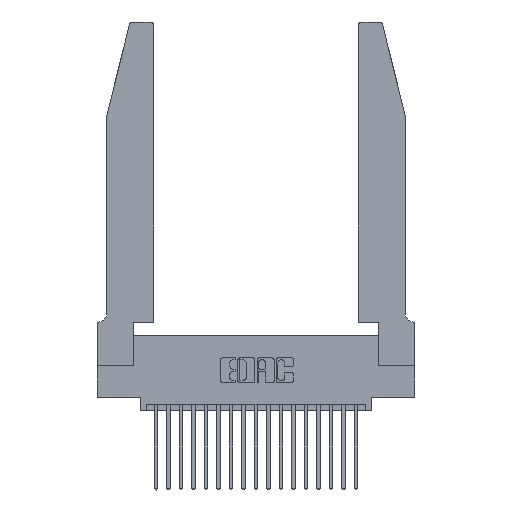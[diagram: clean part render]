
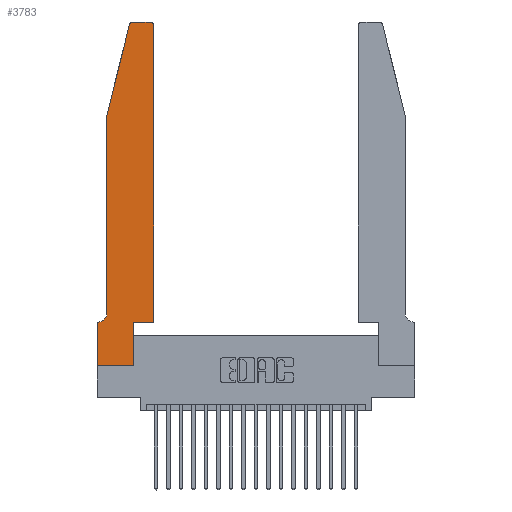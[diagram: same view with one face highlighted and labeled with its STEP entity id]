
A CAD part, top view. The second image highlights one B-rep face of the part: STEP entity #3783.
In plain terms, the highlighted planar face has unit normal (0, 0, 1).
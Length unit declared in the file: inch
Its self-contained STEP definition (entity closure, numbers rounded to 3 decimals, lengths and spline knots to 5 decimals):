
#134 = LINE ( 'NONE', #13619, #5119 ) ;
#401 = VECTOR ( 'NONE', #16446, 39.37008 ) ;
#693 = DIRECTION ( 'NONE',  ( 0., 0., 1. ) ) ;
#990 = LINE ( 'NONE', #7493, #9300 ) ;
#1028 = ORIENTED_EDGE ( 'NONE', *, *, #19197, .T. ) ;
#1058 = DIRECTION ( 'NONE',  ( 0., 0., 1. ) ) ;
#1126 = CARTESIAN_POINT ( 'NONE',  ( 0.284, 2.72, 0.37 ) ) ;
#1162 = VERTEX_POINT ( 'NONE', #3119 ) ;
#1620 = VERTEX_POINT ( 'NONE', #6590 ) ;
#1641 = AXIS2_PLACEMENT_3D ( 'NONE', #12699, #9183, #12479 ) ;
#1657 = CARTESIAN_POINT ( 'NONE',  ( 0., 0.35, 0.37 ) ) ;
#1694 = CARTESIAN_POINT ( 'NONE',  ( 0.25487, 2.72718, 0.37 ) ) ;
#1742 = ORIENTED_EDGE ( 'NONE', *, *, #15930, .T. ) ;
#1983 = CARTESIAN_POINT ( 'NONE',  ( 0., 0., 0.37 ) ) ;
#2002 = CARTESIAN_POINT ( 'NONE',  ( 0.2865, 0., 0.37 ) ) ;
#2012 = CARTESIAN_POINT ( 'NONE',  ( 0.4505, 2.72, 0.37 ) ) ;
#2058 = VECTOR ( 'NONE', #16751, 39.37008 ) ;
#2405 = ORIENTED_EDGE ( 'NONE', *, *, #2979, .T. ) ;
#2886 = CARTESIAN_POINT ( 'NONE',  ( 0.0755, 2., 0.37 ) ) ;
#2979 = EDGE_CURVE ( 'NONE', #1620, #12954, #12759, .T. ) ;
#3119 = CARTESIAN_POINT ( 'NONE',  ( 0.284, 2.75, 0.37 ) ) ;
#3325 = CARTESIAN_POINT ( 'NONE',  ( 0.4505, 0.35, 0.37 ) ) ;
#3480 = EDGE_LOOP ( 'NONE', ( #21405, #15830, #7246, #17913, #7006, #1742, #10078, #2405, #1028, #13669, #14491, #6155 ) ) ;
#3681 = CARTESIAN_POINT ( 'NONE',  ( 0., 0.35, 0.37 ) ) ;
#3783 = ADVANCED_FACE ( 'NONE', ( #17398 ), #11643, .T. ) ;
#3919 = DIRECTION ( 'NONE',  ( 0., 1., 0. ) ) ;
#4017 = CIRCLE ( 'NONE', #12857, 0.03 ) ;
#4219 = VECTOR ( 'NONE', #8856, 39.37008 ) ;
#4847 = LINE ( 'NONE', #3325, #401 ) ;
#5119 = VECTOR ( 'NONE', #16963, 39.37008 ) ;
#5448 = CARTESIAN_POINT ( 'NONE',  ( 0.0755, 0.35, 0.37 ) ) ;
#5594 = EDGE_CURVE ( 'NONE', #10053, #16858, #4847, .T. ) ;
#5713 = VECTOR ( 'NONE', #9882, 39.37008 ) ;
#6047 = DIRECTION ( 'NONE',  ( 1., 0., 0. ) ) ;
#6155 = ORIENTED_EDGE ( 'NONE', *, *, #10545, .T. ) ;
#6590 = CARTESIAN_POINT ( 'NONE',  ( 0., 0., 0.37 ) ) ;
#6824 = CARTESIAN_POINT ( 'NONE',  ( 0.0755, 0.42, 0.37 ) ) ;
#7006 = ORIENTED_EDGE ( 'NONE', *, *, #17472, .T. ) ;
#7246 = ORIENTED_EDGE ( 'NONE', *, *, #12771, .T. ) ;
#7493 = CARTESIAN_POINT ( 'NONE',  ( 0.2865, 0.35, 0.37 ) ) ;
#8364 = VECTOR ( 'NONE', #18694, 39.37008 ) ;
#8472 = CARTESIAN_POINT ( 'NONE',  ( 0.0755, 2., 0.37 ) ) ;
#8676 = EDGE_CURVE ( 'NONE', #1162, #13931, #4017, .T. ) ;
#8788 = LINE ( 'NONE', #17336, #15560 ) ;
#8856 = DIRECTION ( 'NONE',  ( -1., 0., 0. ) ) ;
#8857 = LINE ( 'NONE', #5448, #4219 ) ;
#9134 = CARTESIAN_POINT ( 'NONE',  ( 0.4505, 0.35, 0.37 ) ) ;
#9183 = DIRECTION ( 'NONE',  ( 0., 0., -1. ) ) ;
#9282 = VERTEX_POINT ( 'NONE', #18276 ) ;
#9300 = VECTOR ( 'NONE', #3919, 39.37008 ) ;
#9857 = CIRCLE ( 'NONE', #1641, 0.07 ) ;
#9882 = DIRECTION ( 'NONE',  ( 0., -1., 0. ) ) ;
#9917 = CIRCLE ( 'NONE', #20012, 0.03 ) ;
#9999 = AXIS2_PLACEMENT_3D ( 'NONE', #1657, #13311, #13385 ) ;
#10053 = VERTEX_POINT ( 'NONE', #9134 ) ;
#10078 = ORIENTED_EDGE ( 'NONE', *, *, #15344, .T. ) ;
#10202 = VERTEX_POINT ( 'NONE', #3681 ) ;
#10545 = EDGE_CURVE ( 'NONE', #16858, #17300, #9917, .T. ) ;
#11002 = CARTESIAN_POINT ( 'NONE',  ( 0.0055, 0.35, 0.37 ) ) ;
#11244 = EDGE_CURVE ( 'NONE', #18060, #12360, #11733, .T. ) ;
#11275 = DIRECTION ( 'NONE',  ( -0.239, -0.971, 0. ) ) ;
#11409 = LINE ( 'NONE', #2886, #15280 ) ;
#11643 = PLANE ( 'NONE',  #9999 ) ;
#11733 = LINE ( 'NONE', #8472, #5713 ) ;
#12360 = VERTEX_POINT ( 'NONE', #6824 ) ;
#12396 = DIRECTION ( 'NONE',  ( 1., 0., 0. ) ) ;
#12423 = CARTESIAN_POINT ( 'NONE',  ( 0.4205, 2.72, 0.37 ) ) ;
#12479 = DIRECTION ( 'NONE',  ( -1., 0., 0. ) ) ;
#12699 = CARTESIAN_POINT ( 'NONE',  ( 0.0055, 0.42, 0.37 ) ) ;
#12759 = LINE ( 'NONE', #20064, #2058 ) ;
#12771 = EDGE_CURVE ( 'NONE', #13931, #18060, #11409, .T. ) ;
#12836 = LINE ( 'NONE', #1983, #8364 ) ;
#12857 = AXIS2_PLACEMENT_3D ( 'NONE', #1126, #1058, #6047 ) ;
#12954 = VERTEX_POINT ( 'NONE', #2002 ) ;
#13311 = DIRECTION ( 'NONE',  ( 0., 0., 1. ) ) ;
#13385 = DIRECTION ( 'NONE',  ( 1., 0., 0. ) ) ;
#13619 = CARTESIAN_POINT ( 'NONE',  ( 0.2605, 2.75, 0.37 ) ) ;
#13669 = ORIENTED_EDGE ( 'NONE', *, *, #17344, .T. ) ;
#13931 = VERTEX_POINT ( 'NONE', #1694 ) ;
#14491 = ORIENTED_EDGE ( 'NONE', *, *, #5594, .T. ) ;
#15280 = VECTOR ( 'NONE', #11275, 39.37008 ) ;
#15344 = EDGE_CURVE ( 'NONE', #10202, #1620, #12836, .T. ) ;
#15560 = VECTOR ( 'NONE', #12396, 39.37008 ) ;
#15656 = CARTESIAN_POINT ( 'NONE',  ( 0.4205, 2.75, 0.37 ) ) ;
#15754 = CARTESIAN_POINT ( 'NONE',  ( 0.0755, 2., 0.37 ) ) ;
#15830 = ORIENTED_EDGE ( 'NONE', *, *, #8676, .T. ) ;
#15930 = EDGE_CURVE ( 'NONE', #19371, #10202, #8857, .T. ) ;
#16446 = DIRECTION ( 'NONE',  ( 0., 1., 0. ) ) ;
#16751 = DIRECTION ( 'NONE',  ( 1., 0., 0. ) ) ;
#16858 = VERTEX_POINT ( 'NONE', #2012 ) ;
#16963 = DIRECTION ( 'NONE',  ( -1., 0., 0. ) ) ;
#17300 = VERTEX_POINT ( 'NONE', #15656 ) ;
#17336 = CARTESIAN_POINT ( 'NONE',  ( 0.4505, 0.35, 0.37 ) ) ;
#17344 = EDGE_CURVE ( 'NONE', #9282, #10053, #8788, .T. ) ;
#17398 = FACE_OUTER_BOUND ( 'NONE', #3480, .T. ) ;
#17472 = EDGE_CURVE ( 'NONE', #12360, #19371, #9857, .T. ) ;
#17913 = ORIENTED_EDGE ( 'NONE', *, *, #11244, .T. ) ;
#18060 = VERTEX_POINT ( 'NONE', #15754 ) ;
#18276 = CARTESIAN_POINT ( 'NONE',  ( 0.2865, 0.35, 0.37 ) ) ;
#18694 = DIRECTION ( 'NONE',  ( 0., -1., 0. ) ) ;
#19051 = EDGE_CURVE ( 'NONE', #17300, #1162, #134, .T. ) ;
#19197 = EDGE_CURVE ( 'NONE', #12954, #9282, #990, .T. ) ;
#19371 = VERTEX_POINT ( 'NONE', #11002 ) ;
#20012 = AXIS2_PLACEMENT_3D ( 'NONE', #12423, #693, #20820 ) ;
#20064 = CARTESIAN_POINT ( 'NONE',  ( 0., 0., 0.37 ) ) ;
#20820 = DIRECTION ( 'NONE',  ( 1., 0., 0. ) ) ;
#21405 = ORIENTED_EDGE ( 'NONE', *, *, #19051, .T. ) ;
